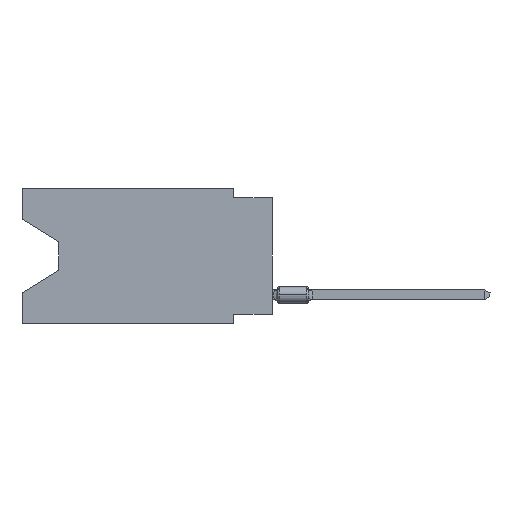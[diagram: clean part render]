
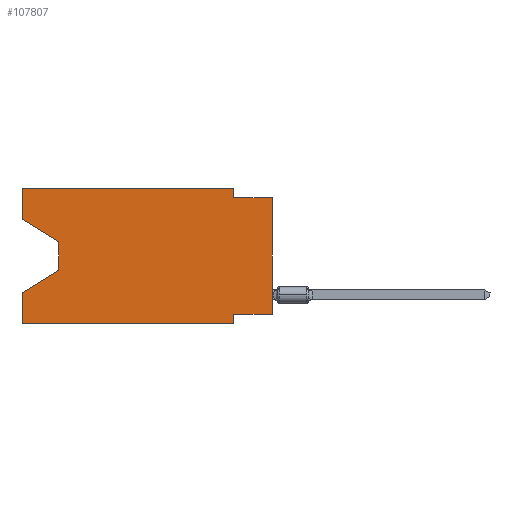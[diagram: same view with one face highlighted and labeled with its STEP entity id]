
A CAD part, left-side view. The second image highlights one B-rep face of the part: STEP entity #107807.
In plain terms, the highlighted planar face has unit normal (-1, 0, 0).
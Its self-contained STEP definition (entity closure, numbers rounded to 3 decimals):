
#5411 = CARTESIAN_POINT ( 'NONE',  ( 0., 16.383, -8.89 ) ) ;
#5927 = LINE ( 'NONE', #7607, #55744 ) ;
#6118 = CARTESIAN_POINT ( 'NONE',  ( 0., 16.383, 0. ) ) ;
#6416 = CARTESIAN_POINT ( 'NONE',  ( 0., 2.54, -8.89 ) ) ;
#7607 = CARTESIAN_POINT ( 'NONE',  ( 0., 13.97, -3.505 ) ) ;
#8735 = VECTOR ( 'NONE', #107786, 1000. ) ;
#8998 = EDGE_LOOP ( 'NONE', ( #37782, #88576, #41742, #59896, #73632, #50476, #61152, #82382, #14514, #94076, #85158, #101568 ) ) ;
#11142 = VECTOR ( 'NONE', #103477, 1000. ) ;
#11214 = LINE ( 'NONE', #55324, #49877 ) ;
#12181 = VERTEX_POINT ( 'NONE', #101047 ) ;
#14514 = ORIENTED_EDGE ( 'NONE', *, *, #86539, .F. ) ;
#15051 = VERTEX_POINT ( 'NONE', #30575 ) ;
#15445 = DIRECTION ( 'NONE',  ( 1., 0., 0. ) ) ;
#15840 = LINE ( 'NONE', #25548, #11142 ) ;
#15904 = EDGE_CURVE ( 'NONE', #15051, #98221, #58344, .T. ) ;
#16557 = LINE ( 'NONE', #51513, #83319 ) ;
#19349 = VECTOR ( 'NONE', #32778, 1000. ) ;
#22191 = CARTESIAN_POINT ( 'NONE',  ( 0., 0., -0.635 ) ) ;
#22231 = CARTESIAN_POINT ( 'NONE',  ( 0., 13.97, -3.505 ) ) ;
#23409 = DIRECTION ( 'NONE',  ( 0., -1., 0. ) ) ;
#25425 = VERTEX_POINT ( 'NONE', #74951 ) ;
#25548 = CARTESIAN_POINT ( 'NONE',  ( 0., 16.383, -8.89 ) ) ;
#30457 = EDGE_CURVE ( 'NONE', #55585, #25425, #75529, .T. ) ;
#30575 = CARTESIAN_POINT ( 'NONE',  ( 0., 0., -8.255 ) ) ;
#32778 = DIRECTION ( 'NONE',  ( 0., 0., -1. ) ) ;
#37782 = ORIENTED_EDGE ( 'NONE', *, *, #54999, .T. ) ;
#38715 = DIRECTION ( 'NONE',  ( 0., 1., 0. ) ) ;
#38865 = DIRECTION ( 'NONE',  ( 0., 0., 1. ) ) ;
#38898 = DIRECTION ( 'NONE',  ( 0., 0., 1. ) ) ;
#41742 = ORIENTED_EDGE ( 'NONE', *, *, #106835, .T. ) ;
#44040 = CARTESIAN_POINT ( 'NONE',  ( 0., 16.383, -6.852 ) ) ;
#47459 = CARTESIAN_POINT ( 'NONE',  ( 0., 16.383, 0. ) ) ;
#48112 = LINE ( 'NONE', #100246, #103174 ) ;
#48523 = LINE ( 'NONE', #75983, #61131 ) ;
#49195 = CARTESIAN_POINT ( 'NONE',  ( 0., 0., 0. ) ) ;
#49877 = VECTOR ( 'NONE', #38715, 1000. ) ;
#50323 = CARTESIAN_POINT ( 'NONE',  ( 0., 16.383, 0. ) ) ;
#50476 = ORIENTED_EDGE ( 'NONE', *, *, #82885, .F. ) ;
#51339 = VERTEX_POINT ( 'NONE', #68023 ) ;
#51415 = CARTESIAN_POINT ( 'NONE',  ( 0., 2.54, -8.255 ) ) ;
#51491 = VERTEX_POINT ( 'NONE', #112692 ) ;
#51513 = CARTESIAN_POINT ( 'NONE',  ( 0., 13.97, -5.385 ) ) ;
#51800 = EDGE_CURVE ( 'NONE', #15051, #110430, #11214, .T. ) ;
#52589 = EDGE_CURVE ( 'NONE', #75967, #70794, #62936, .T. ) ;
#54999 = EDGE_CURVE ( 'NONE', #51339, #108184, #107224, .T. ) ;
#55324 = CARTESIAN_POINT ( 'NONE',  ( 0., 0., -8.255 ) ) ;
#55585 = VERTEX_POINT ( 'NONE', #6118 ) ;
#55744 = VECTOR ( 'NONE', #75804, 1000. ) ;
#57130 = DIRECTION ( 'NONE',  ( 0., -1., 0. ) ) ;
#58245 = DIRECTION ( 'NONE',  ( 0., 0., 1. ) ) ;
#58344 = LINE ( 'NONE', #49195, #76801 ) ;
#58995 = DIRECTION ( 'NONE',  ( 0., 0., -1. ) ) ;
#59672 = AXIS2_PLACEMENT_3D ( 'NONE', #67589, #15445, #58995 ) ;
#59896 = ORIENTED_EDGE ( 'NONE', *, *, #52589, .F. ) ;
#61131 = VECTOR ( 'NONE', #58245, 1000. ) ;
#61152 = ORIENTED_EDGE ( 'NONE', *, *, #51800, .F. ) ;
#62936 = LINE ( 'NONE', #47459, #74732 ) ;
#63429 = EDGE_CURVE ( 'NONE', #25425, #75822, #48112, .T. ) ;
#67589 = CARTESIAN_POINT ( 'NONE',  ( 0., 16.383, 0. ) ) ;
#68023 = CARTESIAN_POINT ( 'NONE',  ( 0., 16.383, -2.038 ) ) ;
#70794 = VERTEX_POINT ( 'NONE', #44040 ) ;
#72720 = VECTOR ( 'NONE', #57130, 1000. ) ;
#73401 = CARTESIAN_POINT ( 'NONE',  ( 0., 16.383, -2.038 ) ) ;
#73632 = ORIENTED_EDGE ( 'NONE', *, *, #90213, .T. ) ;
#74732 = VECTOR ( 'NONE', #38865, 1000. ) ;
#74951 = CARTESIAN_POINT ( 'NONE',  ( 0., 2.54, 0. ) ) ;
#75529 = LINE ( 'NONE', #50323, #98668 ) ;
#75804 = DIRECTION ( 'NONE',  ( 0., 0., -1. ) ) ;
#75822 = VERTEX_POINT ( 'NONE', #98259 ) ;
#75967 = VERTEX_POINT ( 'NONE', #5411 ) ;
#75983 = CARTESIAN_POINT ( 'NONE',  ( 0., 16.383, 0. ) ) ;
#76801 = VECTOR ( 'NONE', #38898, 1000. ) ;
#82382 = ORIENTED_EDGE ( 'NONE', *, *, #15904, .T. ) ;
#82885 = EDGE_CURVE ( 'NONE', #110430, #51491, #84887, .T. ) ;
#83043 = DIRECTION ( 'NONE',  ( 0., 0., -1. ) ) ;
#83319 = VECTOR ( 'NONE', #86444, 1000. ) ;
#84773 = FACE_OUTER_BOUND ( 'NONE', #8998, .T. ) ;
#84887 = LINE ( 'NONE', #6416, #19349 ) ;
#85158 = ORIENTED_EDGE ( 'NONE', *, *, #30457, .F. ) ;
#86444 = DIRECTION ( 'NONE',  ( 0., 0.855, -0.519 ) ) ;
#86539 = EDGE_CURVE ( 'NONE', #75822, #98221, #92638, .T. ) ;
#88576 = ORIENTED_EDGE ( 'NONE', *, *, #99838, .T. ) ;
#90213 = EDGE_CURVE ( 'NONE', #75967, #51491, #15840, .T. ) ;
#92401 = CARTESIAN_POINT ( 'NONE',  ( 0., 0., -0.635 ) ) ;
#92638 = LINE ( 'NONE', #22191, #72720 ) ;
#92639 = EDGE_CURVE ( 'NONE', #51339, #55585, #48523, .T. ) ;
#94076 = ORIENTED_EDGE ( 'NONE', *, *, #63429, .F. ) ;
#98221 = VERTEX_POINT ( 'NONE', #92401 ) ;
#98259 = CARTESIAN_POINT ( 'NONE',  ( 0., 2.54, -0.635 ) ) ;
#98668 = VECTOR ( 'NONE', #23409, 1000. ) ;
#99838 = EDGE_CURVE ( 'NONE', #108184, #12181, #5927, .T. ) ;
#100246 = CARTESIAN_POINT ( 'NONE',  ( 0., 2.54, 0. ) ) ;
#101047 = CARTESIAN_POINT ( 'NONE',  ( 0., 13.97, -5.385 ) ) ;
#101568 = ORIENTED_EDGE ( 'NONE', *, *, #92639, .F. ) ;
#101987 = PLANE ( 'NONE',  #59672 ) ;
#103174 = VECTOR ( 'NONE', #83043, 1000. ) ;
#103477 = DIRECTION ( 'NONE',  ( 0., -1., 0. ) ) ;
#106835 = EDGE_CURVE ( 'NONE', #12181, #70794, #16557, .T. ) ;
#107224 = LINE ( 'NONE', #73401, #8735 ) ;
#107786 = DIRECTION ( 'NONE',  ( 0., -0.855, -0.519 ) ) ;
#107807 = ADVANCED_FACE ( 'NONE', ( #84773 ), #101987, .F. ) ;
#108184 = VERTEX_POINT ( 'NONE', #22231 ) ;
#110430 = VERTEX_POINT ( 'NONE', #51415 ) ;
#112692 = CARTESIAN_POINT ( 'NONE',  ( 0., 2.54, -8.89 ) ) ;
